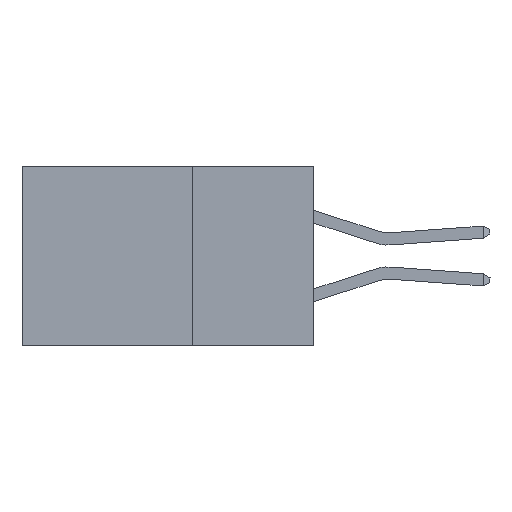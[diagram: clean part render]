
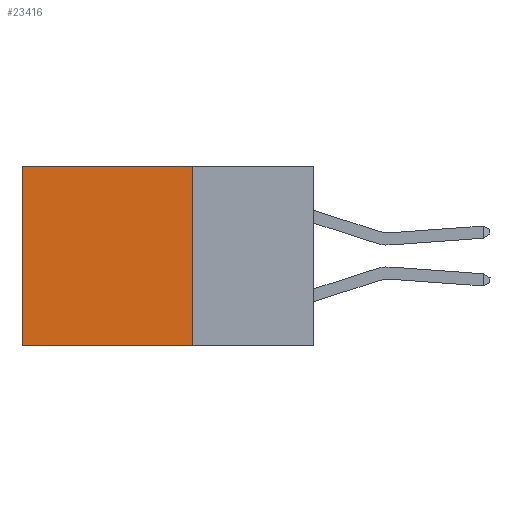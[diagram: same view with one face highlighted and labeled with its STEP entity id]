
A CAD part, left-side view. The second image highlights one B-rep face of the part: STEP entity #23416.
In plain terms, the highlighted planar face has unit normal (-1, 0, 0).
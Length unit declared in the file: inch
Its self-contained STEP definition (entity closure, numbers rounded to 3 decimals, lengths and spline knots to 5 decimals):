
#521 = VERTEX_POINT ( 'NONE', #15463 ) ;
#1602 = DIRECTION ( 'NONE',  ( 0., 1., 0. ) ) ;
#2282 = LINE ( 'NONE', #3283, #17755 ) ;
#3283 = CARTESIAN_POINT ( 'NONE',  ( 0.2875, 0.25, 0. ) ) ;
#3803 = CARTESIAN_POINT ( 'NONE',  ( 0.2875, 0.25, -0.37 ) ) ;
#4194 = VECTOR ( 'NONE', #4909, 39.37008 ) ;
#4238 = PLANE ( 'NONE',  #18526 ) ;
#4909 = DIRECTION ( 'NONE',  ( 0., 0., -1. ) ) ;
#6865 = CARTESIAN_POINT ( 'NONE',  ( 0.2875, 0.25, 0. ) ) ;
#7124 = ORIENTED_EDGE ( 'NONE', *, *, #11537, .T. ) ;
#8839 = CARTESIAN_POINT ( 'NONE',  ( 0.2875, 0.25, 0. ) ) ;
#10333 = DIRECTION ( 'NONE',  ( 0., 0., -1. ) ) ;
#10434 = VERTEX_POINT ( 'NONE', #6865 ) ;
#10461 = VECTOR ( 'NONE', #10333, 39.37008 ) ;
#11537 = EDGE_CURVE ( 'NONE', #521, #20694, #16155, .T. ) ;
#11904 = LINE ( 'NONE', #15605, #4194 ) ;
#11984 = ORIENTED_EDGE ( 'NONE', *, *, #21253, .T. ) ;
#12198 = EDGE_LOOP ( 'NONE', ( #7124, #25840, #12864, #11984 ) ) ;
#12860 = DIRECTION ( 'NONE',  ( 1., 0., 0. ) ) ;
#12864 = ORIENTED_EDGE ( 'NONE', *, *, #20022, .F. ) ;
#13592 = VECTOR ( 'NONE', #19014, 39.37008 ) ;
#13761 = CARTESIAN_POINT ( 'NONE',  ( 0.2875, 0.25, -0.37 ) ) ;
#14368 = EDGE_CURVE ( 'NONE', #26046, #20694, #22939, .T. ) ;
#14836 = CARTESIAN_POINT ( 'NONE',  ( 0.2875, 0.6, 0. ) ) ;
#15463 = CARTESIAN_POINT ( 'NONE',  ( 0.2875, 0.6, 0. ) ) ;
#15605 = CARTESIAN_POINT ( 'NONE',  ( 0.2875, 0.25, 0. ) ) ;
#16155 = LINE ( 'NONE', #14836, #10461 ) ;
#16645 = FACE_OUTER_BOUND ( 'NONE', #12198, .T. ) ;
#17755 = VECTOR ( 'NONE', #1602, 39.37008 ) ;
#18526 = AXIS2_PLACEMENT_3D ( 'NONE', #8839, #12860, #19252 ) ;
#19014 = DIRECTION ( 'NONE',  ( 0., 1., 0. ) ) ;
#19252 = DIRECTION ( 'NONE',  ( 0., 0., -1. ) ) ;
#20022 = EDGE_CURVE ( 'NONE', #10434, #26046, #11904, .T. ) ;
#20694 = VERTEX_POINT ( 'NONE', #21344 ) ;
#21253 = EDGE_CURVE ( 'NONE', #10434, #521, #2282, .T. ) ;
#21344 = CARTESIAN_POINT ( 'NONE',  ( 0.2875, 0.6, -0.37 ) ) ;
#22939 = LINE ( 'NONE', #3803, #13592 ) ;
#23416 = ADVANCED_FACE ( 'NONE', ( #16645 ), #4238, .F. ) ;
#25840 = ORIENTED_EDGE ( 'NONE', *, *, #14368, .F. ) ;
#26046 = VERTEX_POINT ( 'NONE', #13761 ) ;
